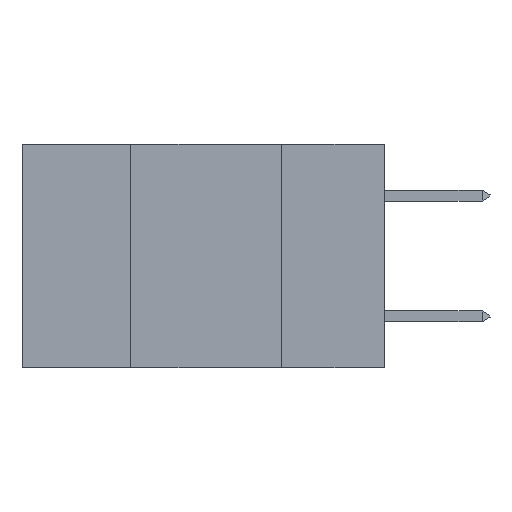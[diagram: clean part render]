
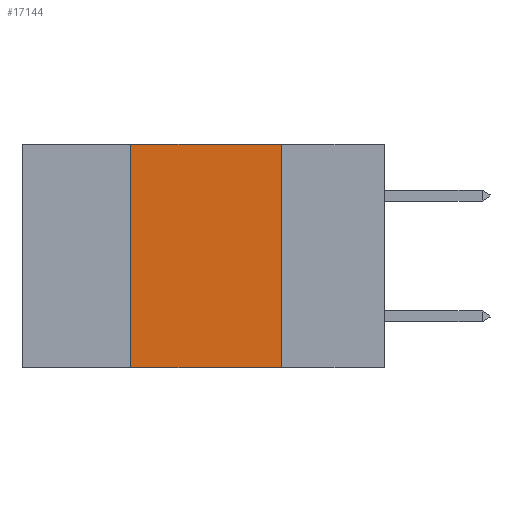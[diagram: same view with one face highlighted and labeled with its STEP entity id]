
A CAD part, left-side view. The second image highlights one B-rep face of the part: STEP entity #17144.
In plain terms, the highlighted planar face has unit normal (-1, 0, 0).
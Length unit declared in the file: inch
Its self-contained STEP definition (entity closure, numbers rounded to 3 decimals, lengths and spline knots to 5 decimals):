
#1190 = ORIENTED_EDGE ( 'NONE', *, *, #8730, .F. ) ;
#1811 = LINE ( 'NONE', #22879, #21212 ) ;
#1939 = AXIS2_PLACEMENT_3D ( 'NONE', #3487, #33710, #27283 ) ;
#2947 = EDGE_CURVE ( 'NONE', #32059, #26327, #17421, .T. ) ;
#3237 = DIRECTION ( 'NONE',  ( 0., 0., -1. ) ) ;
#3487 = CARTESIAN_POINT ( 'NONE',  ( 0., 0.6, 0. ) ) ;
#6279 = PLANE ( 'NONE',  #1939 ) ;
#8730 = EDGE_CURVE ( 'NONE', #14420, #32059, #1811, .T. ) ;
#9595 = CARTESIAN_POINT ( 'NONE',  ( 0., 0.42, -0.37 ) ) ;
#11422 = ORIENTED_EDGE ( 'NONE', *, *, #12111, .T. ) ;
#12111 = EDGE_CURVE ( 'NONE', #14420, #19297, #21619, .T. ) ;
#13298 = EDGE_LOOP ( 'NONE', ( #22898, #23639, #1190, #11422 ) ) ;
#14420 = VERTEX_POINT ( 'NONE', #9595 ) ;
#15730 = FACE_OUTER_BOUND ( 'NONE', #13298, .T. ) ;
#17144 = ADVANCED_FACE ( 'NONE', ( #15730 ), #6279, .F. ) ;
#17421 = LINE ( 'NONE', #32217, #20284 ) ;
#17686 = CARTESIAN_POINT ( 'NONE',  ( 0., 0.17, -0.37 ) ) ;
#18443 = CARTESIAN_POINT ( 'NONE',  ( 0., 0.17, 0. ) ) ;
#19297 = VERTEX_POINT ( 'NONE', #17686 ) ;
#19300 = CARTESIAN_POINT ( 'NONE',  ( 0., 0.6, -0.37 ) ) ;
#20284 = VECTOR ( 'NONE', #35260, 39.37008 ) ;
#21212 = VECTOR ( 'NONE', #38161, 39.37008 ) ;
#21619 = LINE ( 'NONE', #19300, #27767 ) ;
#21815 = LINE ( 'NONE', #18443, #26534 ) ;
#22879 = CARTESIAN_POINT ( 'NONE',  ( 0., 0.42, 0. ) ) ;
#22898 = ORIENTED_EDGE ( 'NONE', *, *, #33845, .F. ) ;
#23639 = ORIENTED_EDGE ( 'NONE', *, *, #2947, .F. ) ;
#26327 = VERTEX_POINT ( 'NONE', #30683 ) ;
#26534 = VECTOR ( 'NONE', #3237, 39.37008 ) ;
#27283 = DIRECTION ( 'NONE',  ( 0., 0., -1. ) ) ;
#27767 = VECTOR ( 'NONE', #28275, 39.37008 ) ;
#28275 = DIRECTION ( 'NONE',  ( 0., -1., 0. ) ) ;
#30683 = CARTESIAN_POINT ( 'NONE',  ( 0., 0.17, 0. ) ) ;
#32059 = VERTEX_POINT ( 'NONE', #32516 ) ;
#32217 = CARTESIAN_POINT ( 'NONE',  ( 0., 0.6, 0. ) ) ;
#32516 = CARTESIAN_POINT ( 'NONE',  ( 0., 0.42, 0. ) ) ;
#33710 = DIRECTION ( 'NONE',  ( 1., 0., 0. ) ) ;
#33845 = EDGE_CURVE ( 'NONE', #26327, #19297, #21815, .T. ) ;
#35260 = DIRECTION ( 'NONE',  ( 0., -1., 0. ) ) ;
#38161 = DIRECTION ( 'NONE',  ( 0., 0., 1. ) ) ;
